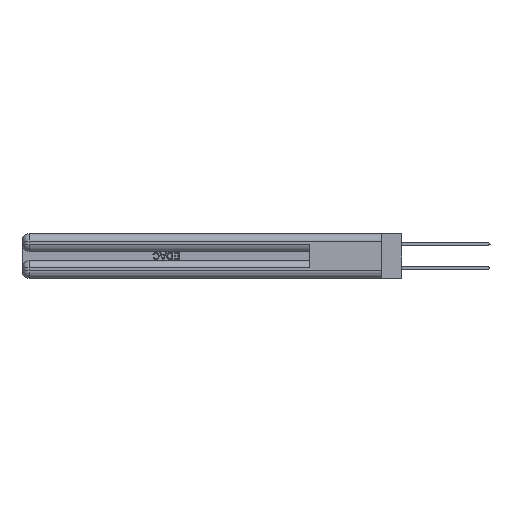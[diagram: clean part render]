
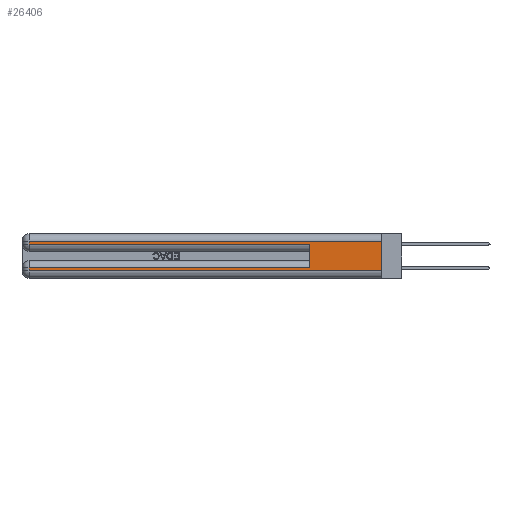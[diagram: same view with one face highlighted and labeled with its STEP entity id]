
A CAD part, left-side view. The second image highlights one B-rep face of the part: STEP entity #26406.
In plain terms, the highlighted planar face has unit normal (-1, 0, 0).
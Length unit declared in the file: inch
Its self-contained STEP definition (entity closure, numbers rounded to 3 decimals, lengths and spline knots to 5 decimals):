
#759 = FACE_OUTER_BOUND ( 'NONE', #39478, .T. ) ;
#1021 = VERTEX_POINT ( 'NONE', #48623 ) ;
#2026 = CARTESIAN_POINT ( 'NONE',  ( 0., 0., 0.085 ) ) ;
#4052 = CARTESIAN_POINT ( 'NONE',  ( 0., 0., 0.285 ) ) ;
#4441 = EDGE_CURVE ( 'NONE', #36990, #26325, #33918, .T. ) ;
#4523 = LINE ( 'NONE', #2026, #23746 ) ;
#4686 = CARTESIAN_POINT ( 'NONE',  ( 0., 0., 0.37 ) ) ;
#5139 = VERTEX_POINT ( 'NONE', #39994 ) ;
#5456 = DIRECTION ( 'NONE',  ( 0., 0., -1. ) ) ;
#7907 = CARTESIAN_POINT ( 'NONE',  ( 0., 2.94, 0.06 ) ) ;
#9085 = VERTEX_POINT ( 'NONE', #25610 ) ;
#9978 = ORIENTED_EDGE ( 'NONE', *, *, #36273, .T. ) ;
#10476 = VERTEX_POINT ( 'NONE', #45567 ) ;
#10771 = LINE ( 'NONE', #15756, #31183 ) ;
#11517 = DIRECTION ( 'NONE',  ( 0., 0., -1. ) ) ;
#12444 = PLANE ( 'NONE',  #16561 ) ;
#13604 = LINE ( 'NONE', #40744, #21393 ) ;
#13894 = DIRECTION ( 'NONE',  ( 0., 1., 0. ) ) ;
#14121 = VERTEX_POINT ( 'NONE', #20078 ) ;
#14383 = LINE ( 'NONE', #30835, #22157 ) ;
#15233 = ORIENTED_EDGE ( 'NONE', *, *, #4441, .T. ) ;
#15607 = VECTOR ( 'NONE', #38097, 39.37008 ) ;
#15756 = CARTESIAN_POINT ( 'NONE',  ( 0., 0., 0.06 ) ) ;
#16300 = DIRECTION ( 'NONE',  ( 0., 0., -1. ) ) ;
#16472 = LINE ( 'NONE', #4052, #48249 ) ;
#16561 = AXIS2_PLACEMENT_3D ( 'NONE', #4686, #39305, #16300 ) ;
#17029 = EDGE_CURVE ( 'NONE', #1021, #14121, #13604, .T. ) ;
#20078 = CARTESIAN_POINT ( 'NONE',  ( 0., 2.94, 0.31 ) ) ;
#20124 = EDGE_CURVE ( 'NONE', #5139, #36990, #4523, .T. ) ;
#21393 = VECTOR ( 'NONE', #13894, 39.37008 ) ;
#22051 = VECTOR ( 'NONE', #11517, 39.37008 ) ;
#22157 = VECTOR ( 'NONE', #34733, 39.37008 ) ;
#23146 = CARTESIAN_POINT ( 'NONE',  ( 0., 0., 0.06 ) ) ;
#23746 = VECTOR ( 'NONE', #40352, 39.37008 ) ;
#25610 = CARTESIAN_POINT ( 'NONE',  ( 0., 2.94, 0.285 ) ) ;
#26325 = VERTEX_POINT ( 'NONE', #7907 ) ;
#26406 = ADVANCED_FACE ( 'NONE', ( #759 ), #12444, .F. ) ;
#26748 = CARTESIAN_POINT ( 'NONE',  ( 0., 2.94, 0.37 ) ) ;
#27046 = DIRECTION ( 'NONE',  ( 0., -1., 0. ) ) ;
#27489 = CARTESIAN_POINT ( 'NONE',  ( 0., 2.94, 0.085 ) ) ;
#28450 = CARTESIAN_POINT ( 'NONE',  ( 0., 2.94, 0.37 ) ) ;
#30835 = CARTESIAN_POINT ( 'NONE',  ( 0., 0., 0.37 ) ) ;
#31183 = VECTOR ( 'NONE', #42578, 39.37008 ) ;
#32289 = LINE ( 'NONE', #26748, #22051 ) ;
#33441 = EDGE_CURVE ( 'NONE', #5139, #10476, #36050, .T. ) ;
#33499 = EDGE_CURVE ( 'NONE', #1021, #40115, #14383, .T. ) ;
#33514 = EDGE_CURVE ( 'NONE', #26325, #40115, #10771, .T. ) ;
#33918 = LINE ( 'NONE', #28450, #35148 ) ;
#34733 = DIRECTION ( 'NONE',  ( 0., 0., -1. ) ) ;
#35148 = VECTOR ( 'NONE', #5456, 39.37008 ) ;
#36050 = LINE ( 'NONE', #49636, #15607 ) ;
#36273 = EDGE_CURVE ( 'NONE', #9085, #10476, #16472, .T. ) ;
#36503 = ORIENTED_EDGE ( 'NONE', *, *, #33441, .F. ) ;
#36990 = VERTEX_POINT ( 'NONE', #27489 ) ;
#37794 = ORIENTED_EDGE ( 'NONE', *, *, #33514, .T. ) ;
#38097 = DIRECTION ( 'NONE',  ( 0., 0., 1. ) ) ;
#39305 = DIRECTION ( 'NONE',  ( 1., 0., 0. ) ) ;
#39478 = EDGE_LOOP ( 'NONE', ( #45601, #43797, #47769, #9978, #36503, #39845, #15233, #37794 ) ) ;
#39845 = ORIENTED_EDGE ( 'NONE', *, *, #20124, .T. ) ;
#39994 = CARTESIAN_POINT ( 'NONE',  ( 0., 0.6, 0.085 ) ) ;
#40115 = VERTEX_POINT ( 'NONE', #23146 ) ;
#40352 = DIRECTION ( 'NONE',  ( 0., 1., 0. ) ) ;
#40744 = CARTESIAN_POINT ( 'NONE',  ( 0., 0., 0.31 ) ) ;
#42578 = DIRECTION ( 'NONE',  ( 0., -1., 0. ) ) ;
#43797 = ORIENTED_EDGE ( 'NONE', *, *, #17029, .T. ) ;
#45567 = CARTESIAN_POINT ( 'NONE',  ( 0., 0.6, 0.285 ) ) ;
#45601 = ORIENTED_EDGE ( 'NONE', *, *, #33499, .F. ) ;
#46738 = EDGE_CURVE ( 'NONE', #14121, #9085, #32289, .T. ) ;
#47769 = ORIENTED_EDGE ( 'NONE', *, *, #46738, .T. ) ;
#48249 = VECTOR ( 'NONE', #27046, 39.37008 ) ;
#48623 = CARTESIAN_POINT ( 'NONE',  ( 0., 0., 0.31 ) ) ;
#49636 = CARTESIAN_POINT ( 'NONE',  ( 0., 0.6, 0.145 ) ) ;
